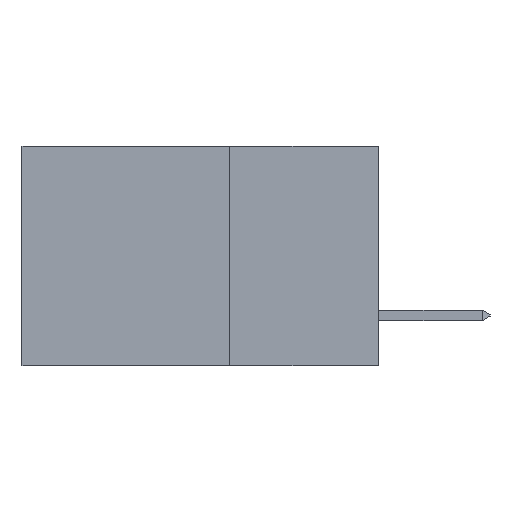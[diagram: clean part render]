
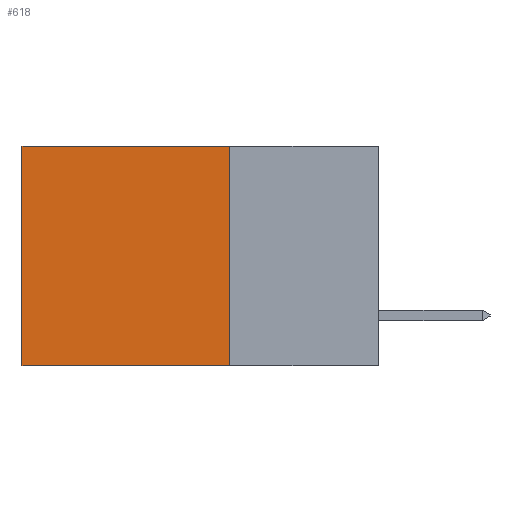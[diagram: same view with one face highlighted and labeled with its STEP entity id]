
A CAD part, left-side view. The second image highlights one B-rep face of the part: STEP entity #618.
In plain terms, the highlighted planar face has unit normal (-1, 0, 0).
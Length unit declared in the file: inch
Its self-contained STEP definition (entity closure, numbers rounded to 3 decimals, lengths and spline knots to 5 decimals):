
#618 = ADVANCED_FACE ( 'NONE', ( #25044 ), #13510, .F. ) ;
#1279 = EDGE_CURVE ( 'NONE', #16240, #10841, #24077, .T. ) ;
#1945 = LINE ( 'NONE', #10955, #13559 ) ;
#2379 = EDGE_CURVE ( 'NONE', #16240, #7581, #12394, .T. ) ;
#2851 = CARTESIAN_POINT ( 'NONE',  ( 0.2615, 0.25, -0.37 ) ) ;
#3740 = EDGE_LOOP ( 'NONE', ( #9676, #21308, #19394, #6925 ) ) ;
#3906 = CARTESIAN_POINT ( 'NONE',  ( 0.2615, 0.25, -0.37 ) ) ;
#4086 = DIRECTION ( 'NONE',  ( 1., 0., 0. ) ) ;
#4946 = VECTOR ( 'NONE', #23114, 39.37008 ) ;
#6925 = ORIENTED_EDGE ( 'NONE', *, *, #1279, .T. ) ;
#7419 = CARTESIAN_POINT ( 'NONE',  ( 0.2615, 0.25, 0. ) ) ;
#7581 = VERTEX_POINT ( 'NONE', #8446 ) ;
#8446 = CARTESIAN_POINT ( 'NONE',  ( 0.2615, 0.25, -0.37 ) ) ;
#9676 = ORIENTED_EDGE ( 'NONE', *, *, #18069, .T. ) ;
#9764 = LINE ( 'NONE', #2851, #4946 ) ;
#9869 = DIRECTION ( 'NONE',  ( 0., 0., -1. ) ) ;
#10841 = VERTEX_POINT ( 'NONE', #14098 ) ;
#10955 = CARTESIAN_POINT ( 'NONE',  ( 0.2615, 0.6, -0.37 ) ) ;
#11675 = CARTESIAN_POINT ( 'NONE',  ( 0.2615, 0.6, -0.37 ) ) ;
#12394 = LINE ( 'NONE', #13008, #13680 ) ;
#12746 = DIRECTION ( 'NONE',  ( 0., 0., -1. ) ) ;
#13008 = CARTESIAN_POINT ( 'NONE',  ( 0.2615, 0.25, -0.37 ) ) ;
#13037 = DIRECTION ( 'NONE',  ( 0., 0., -1. ) ) ;
#13421 = VECTOR ( 'NONE', #23749, 39.37008 ) ;
#13510 = PLANE ( 'NONE',  #21727 ) ;
#13559 = VECTOR ( 'NONE', #13037, 39.37008 ) ;
#13680 = VECTOR ( 'NONE', #12746, 39.37008 ) ;
#14098 = CARTESIAN_POINT ( 'NONE',  ( 0.2615, 0.6, 0. ) ) ;
#16240 = VERTEX_POINT ( 'NONE', #7419 ) ;
#16276 = VERTEX_POINT ( 'NONE', #11675 ) ;
#18069 = EDGE_CURVE ( 'NONE', #10841, #16276, #1945, .T. ) ;
#19394 = ORIENTED_EDGE ( 'NONE', *, *, #2379, .F. ) ;
#21262 = EDGE_CURVE ( 'NONE', #7581, #16276, #9764, .T. ) ;
#21308 = ORIENTED_EDGE ( 'NONE', *, *, #21262, .F. ) ;
#21727 = AXIS2_PLACEMENT_3D ( 'NONE', #3906, #4086, #9869 ) ;
#23114 = DIRECTION ( 'NONE',  ( 0., 1., 0. ) ) ;
#23749 = DIRECTION ( 'NONE',  ( 0., 1., 0. ) ) ;
#24077 = LINE ( 'NONE', #24394, #13421 ) ;
#24394 = CARTESIAN_POINT ( 'NONE',  ( 0.2615, 0.25, 0. ) ) ;
#25044 = FACE_OUTER_BOUND ( 'NONE', #3740, .T. ) ;
